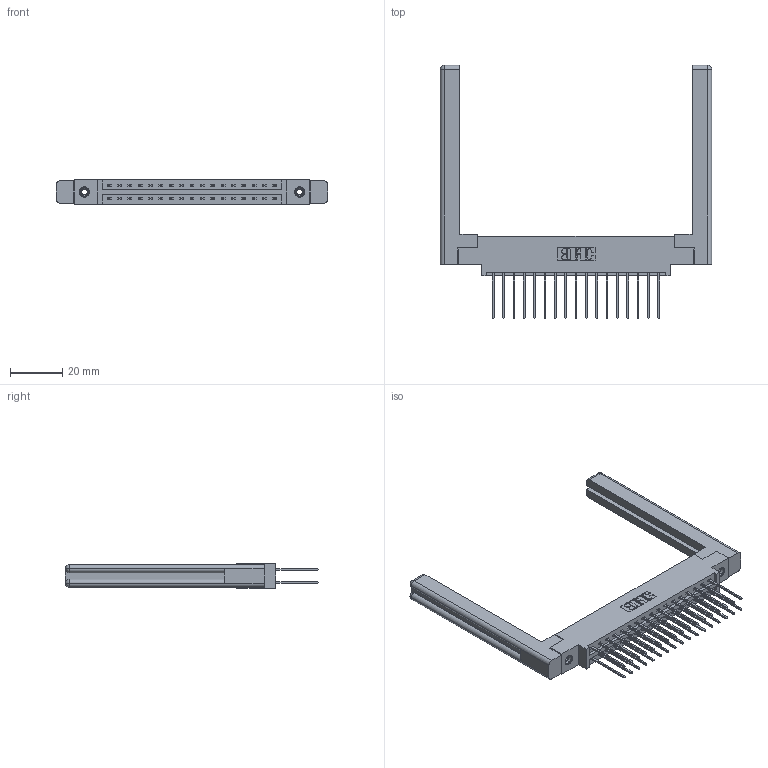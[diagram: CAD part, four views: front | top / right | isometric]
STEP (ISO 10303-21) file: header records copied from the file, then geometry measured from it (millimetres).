
FILE_DESCRIPTION (( 'STEP AP203' ), '1' );
FILE_NAME ('337-034-542-858.STEP', '2019-10-11T02:04:21', ( '' ), ( '' ), 'SwSTEP 2.0', 'SolidWorks 2016', '' );
FILE_SCHEMA (( 'CONFIG_CONTROL_DESIGN' ));
Length unit declared in the file: inch
Products named in the file (5): 345-250-001_345-250-001-102; 307-220-058; 337-034-542-858; 345-292-001_345-293-142; 337 Part_0.170 Offset - 0.156 Dia-TI
Assembly tree (39 placements, depth 2):
  337-034-542-858
    337 Part_0.170 Offset - 0.156 Dia-TI
    345-292-001_345-293-142  x34
    345-250-001_345-250-001-102  x2
    307-220-058  x2
Bounding box: 103.99 x 97.03 x 9.4 mm (x, y, z)
Volume: 17809.6 mm3; surface area: 17761.2 mm2
Topology: 39 solids, 39 shells, 2096 faces, 6151 edges, 4042 vertices
Faces by surface type: plane 1450, cylinder 622, cone 12, torus 12
Entity records: 19198 total; most frequent: CARTESIAN_POINT 3265, ORIENTED_EDGE 3140, DIRECTION 2838, EDGE_CURVE 1570, VECTOR 1394, LINE 1394, VERTEX_POINT 1038, AXIS2_PLACEMENT_3D 722
